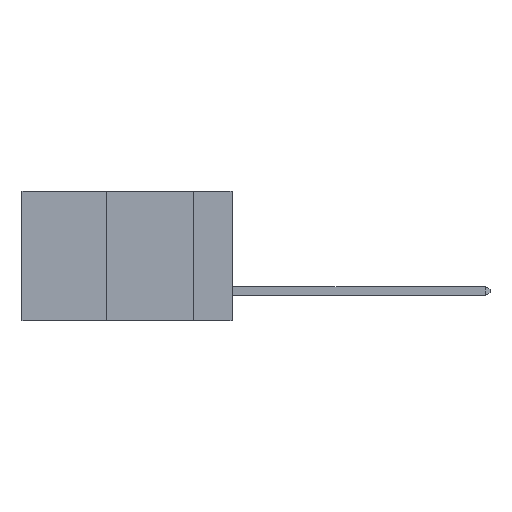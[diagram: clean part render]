
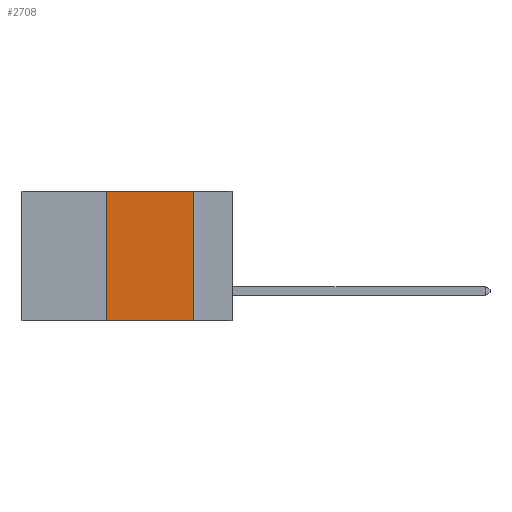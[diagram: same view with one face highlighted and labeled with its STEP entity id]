
A CAD part, left-side view. The second image highlights one B-rep face of the part: STEP entity #2708.
In plain terms, the highlighted planar face has unit normal (-1, 0, 0).
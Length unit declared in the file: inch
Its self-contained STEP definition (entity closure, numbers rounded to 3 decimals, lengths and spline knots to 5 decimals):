
#1222 = CARTESIAN_POINT ( 'NONE',  ( 0., 0.11, -0.37 ) ) ;
#1411 = DIRECTION ( 'NONE',  ( 0., 0., -1. ) ) ;
#2161 = DIRECTION ( 'NONE',  ( 0., 0., -1. ) ) ;
#2465 = VERTEX_POINT ( 'NONE', #5550 ) ;
#2708 = ADVANCED_FACE ( 'NONE', ( #19056 ), #7560, .F. ) ;
#3960 = DIRECTION ( 'NONE',  ( 1., 0., 0. ) ) ;
#4306 = LINE ( 'NONE', #15463, #11692 ) ;
#4727 = EDGE_CURVE ( 'NONE', #2465, #14000, #11729, .T. ) ;
#4825 = VECTOR ( 'NONE', #18149, 39.37008 ) ;
#4964 = CARTESIAN_POINT ( 'NONE',  ( 0., 0.36, 0. ) ) ;
#5305 = ORIENTED_EDGE ( 'NONE', *, *, #4727, .F. ) ;
#5361 = ORIENTED_EDGE ( 'NONE', *, *, #16437, .F. ) ;
#5550 = CARTESIAN_POINT ( 'NONE',  ( 0., 0.36, 0. ) ) ;
#6154 = ORIENTED_EDGE ( 'NONE', *, *, #13483, .T. ) ;
#7560 = PLANE ( 'NONE',  #9874 ) ;
#8079 = LINE ( 'NONE', #9599, #11487 ) ;
#8745 = LINE ( 'NONE', #4964, #4825 ) ;
#9131 = ORIENTED_EDGE ( 'NONE', *, *, #12893, .F. ) ;
#9599 = CARTESIAN_POINT ( 'NONE',  ( 0., 0.11, 0. ) ) ;
#9874 = AXIS2_PLACEMENT_3D ( 'NONE', #14900, #3960, #1411 ) ;
#11487 = VECTOR ( 'NONE', #2161, 39.37008 ) ;
#11692 = VECTOR ( 'NONE', #16932, 39.37008 ) ;
#11729 = LINE ( 'NONE', #17212, #15154 ) ;
#12893 = EDGE_CURVE ( 'NONE', #14000, #13129, #8079, .T. ) ;
#13058 = CARTESIAN_POINT ( 'NONE',  ( 0., 0.36, -0.37 ) ) ;
#13129 = VERTEX_POINT ( 'NONE', #1222 ) ;
#13483 = EDGE_CURVE ( 'NONE', #18787, #13129, #4306, .T. ) ;
#14000 = VERTEX_POINT ( 'NONE', #16534 ) ;
#14900 = CARTESIAN_POINT ( 'NONE',  ( 0., 0.6, 0. ) ) ;
#15154 = VECTOR ( 'NONE', #18274, 39.37008 ) ;
#15463 = CARTESIAN_POINT ( 'NONE',  ( 0., 0.6, -0.37 ) ) ;
#16115 = EDGE_LOOP ( 'NONE', ( #9131, #5305, #5361, #6154 ) ) ;
#16437 = EDGE_CURVE ( 'NONE', #18787, #2465, #8745, .T. ) ;
#16534 = CARTESIAN_POINT ( 'NONE',  ( 0., 0.11, 0. ) ) ;
#16932 = DIRECTION ( 'NONE',  ( 0., -1., 0. ) ) ;
#17212 = CARTESIAN_POINT ( 'NONE',  ( 0., 0.6, 0. ) ) ;
#18149 = DIRECTION ( 'NONE',  ( 0., 0., 1. ) ) ;
#18274 = DIRECTION ( 'NONE',  ( 0., -1., 0. ) ) ;
#18787 = VERTEX_POINT ( 'NONE', #13058 ) ;
#19056 = FACE_OUTER_BOUND ( 'NONE', #16115, .T. ) ;
